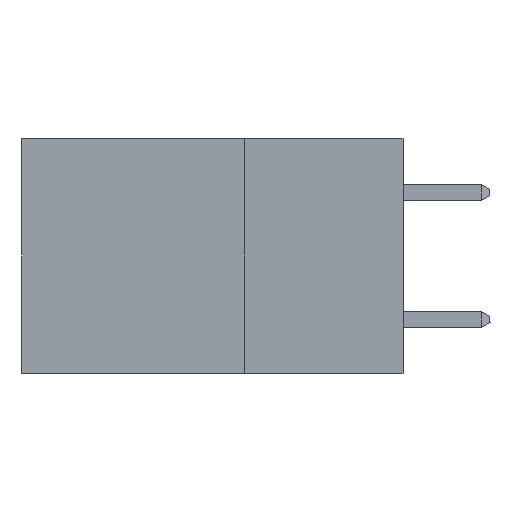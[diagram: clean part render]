
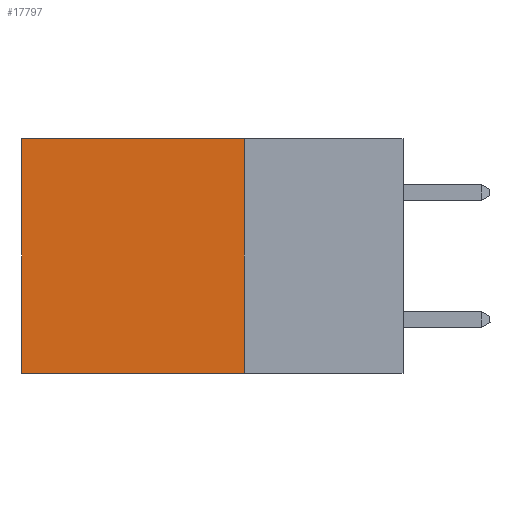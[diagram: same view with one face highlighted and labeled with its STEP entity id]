
A CAD part, left-side view. The second image highlights one B-rep face of the part: STEP entity #17797.
In plain terms, the highlighted planar face has unit normal (-1, 0, 0).
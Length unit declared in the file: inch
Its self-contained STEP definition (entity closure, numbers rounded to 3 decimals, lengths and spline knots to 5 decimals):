
#545 = EDGE_LOOP ( 'NONE', ( #19542, #17222, #2867, #5863 ) ) ;
#769 = VERTEX_POINT ( 'NONE', #17955 ) ;
#886 = DIRECTION ( 'NONE',  ( 0., 0., -1. ) ) ;
#1190 = EDGE_CURVE ( 'NONE', #15036, #769, #18214, .T. ) ;
#1330 = AXIS2_PLACEMENT_3D ( 'NONE', #5056, #20162, #10098 ) ;
#2732 = DIRECTION ( 'NONE',  ( 0., 1., 0. ) ) ;
#2867 = ORIENTED_EDGE ( 'NONE', *, *, #21498, .F. ) ;
#2911 = VECTOR ( 'NONE', #7278, 39.37008 ) ;
#4930 = VERTEX_POINT ( 'NONE', #15256 ) ;
#5056 = CARTESIAN_POINT ( 'NONE',  ( 0.2875, 0.25, 0. ) ) ;
#5863 = ORIENTED_EDGE ( 'NONE', *, *, #15271, .T. ) ;
#6834 = FACE_OUTER_BOUND ( 'NONE', #545, .T. ) ;
#7278 = DIRECTION ( 'NONE',  ( 0., 0., -1. ) ) ;
#8115 = VERTEX_POINT ( 'NONE', #11435 ) ;
#8385 = PLANE ( 'NONE',  #1330 ) ;
#8681 = VECTOR ( 'NONE', #2732, 39.37008 ) ;
#10098 = DIRECTION ( 'NONE',  ( 0., 0., -1. ) ) ;
#10813 = EDGE_CURVE ( 'NONE', #8115, #769, #20070, .T. ) ;
#11435 = CARTESIAN_POINT ( 'NONE',  ( 0.2875, 0.6, 0. ) ) ;
#12742 = CARTESIAN_POINT ( 'NONE',  ( 0.2875, 0.6, 0. ) ) ;
#13119 = CARTESIAN_POINT ( 'NONE',  ( 0.2875, 0.25, 0. ) ) ;
#14534 = CARTESIAN_POINT ( 'NONE',  ( 0.2875, 0.25, -0.37 ) ) ;
#14796 = DIRECTION ( 'NONE',  ( 0., 1., 0. ) ) ;
#15036 = VERTEX_POINT ( 'NONE', #17493 ) ;
#15256 = CARTESIAN_POINT ( 'NONE',  ( 0.2875, 0.25, 0. ) ) ;
#15271 = EDGE_CURVE ( 'NONE', #4930, #8115, #21657, .T. ) ;
#15838 = LINE ( 'NONE', #19075, #2911 ) ;
#17222 = ORIENTED_EDGE ( 'NONE', *, *, #1190, .F. ) ;
#17493 = CARTESIAN_POINT ( 'NONE',  ( 0.2875, 0.25, -0.37 ) ) ;
#17771 = VECTOR ( 'NONE', #14796, 39.37008 ) ;
#17797 = ADVANCED_FACE ( 'NONE', ( #6834 ), #8385, .F. ) ;
#17955 = CARTESIAN_POINT ( 'NONE',  ( 0.2875, 0.6, -0.37 ) ) ;
#18214 = LINE ( 'NONE', #14534, #8681 ) ;
#18512 = VECTOR ( 'NONE', #886, 39.37008 ) ;
#19075 = CARTESIAN_POINT ( 'NONE',  ( 0.2875, 0.25, 0. ) ) ;
#19542 = ORIENTED_EDGE ( 'NONE', *, *, #10813, .T. ) ;
#20070 = LINE ( 'NONE', #12742, #18512 ) ;
#20162 = DIRECTION ( 'NONE',  ( 1., 0., 0. ) ) ;
#21498 = EDGE_CURVE ( 'NONE', #4930, #15036, #15838, .T. ) ;
#21657 = LINE ( 'NONE', #13119, #17771 ) ;
